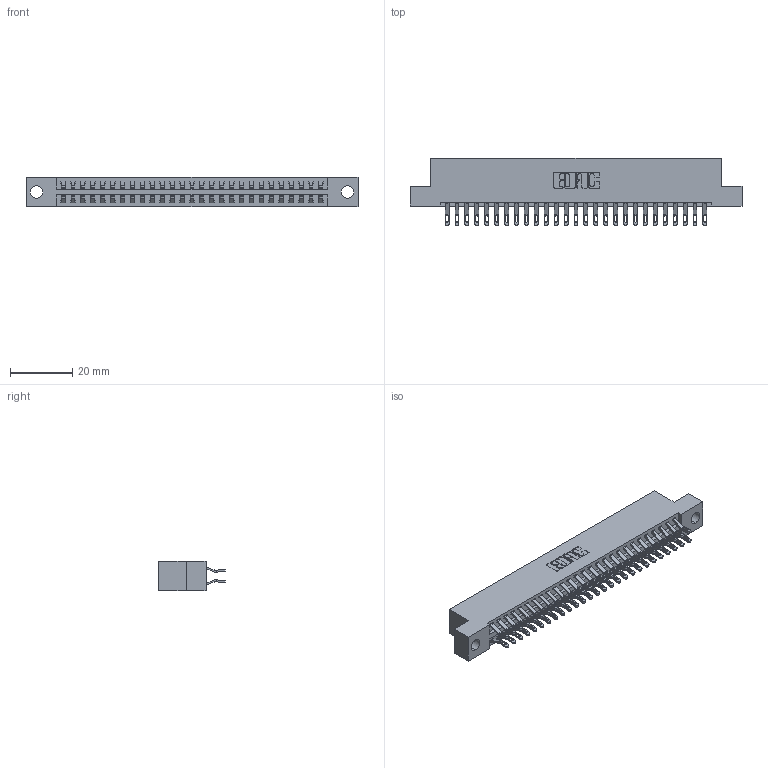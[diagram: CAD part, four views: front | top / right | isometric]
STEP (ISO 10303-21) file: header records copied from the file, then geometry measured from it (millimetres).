
FILE_DESCRIPTION (( 'STEP AP203' ), '1' );
FILE_NAME ('346-054-555-204.STEP', '2022-05-21T03:48:33', ( '' ), ( '' ), 'SwSTEP 2.0', 'SolidWorks 2020', '' );
FILE_SCHEMA (( 'CONFIG_CONTROL_DESIGN' ));
Length unit declared in the file: inch
Products named in the file (3): 346 Part_Flush Mounting Lugs - 0.156 Dia-TH; 345-292-001_555 Tail; 346-054-555-204
Assembly tree (55 placements, depth 2):
  346-054-555-204
    346 Part_Flush Mounting Lugs - 0.156 Dia-TH
    345-292-001_555 Tail  x54
Bounding box: 106.3 x 21.46 x 9.4 mm (x, y, z)
Volume: 10299.6 mm3; surface area: 14328 mm2
Topology: 55 solids, 55 shells, 3268 faces, 10247 edges, 6830 vertices
Faces by surface type: plane 1872, cylinder 1396
Entity records: 20385 total; most frequent: CARTESIAN_POINT 3420, ORIENTED_EDGE 3322, DIRECTION 3033, EDGE_CURVE 1661, LINE 1401, VECTOR 1401, VERTEX_POINT 1106, AXIS2_PLACEMENT_3D 816
